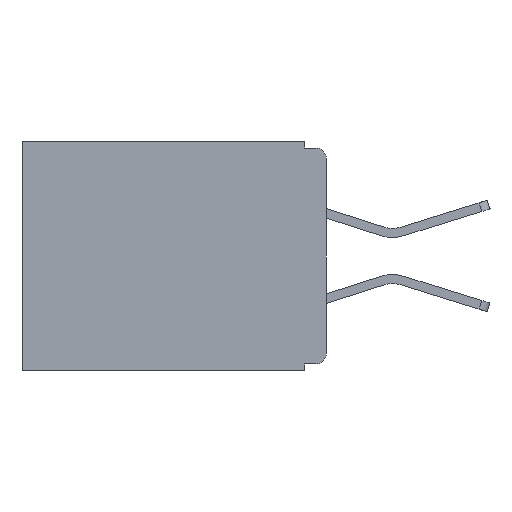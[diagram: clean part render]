
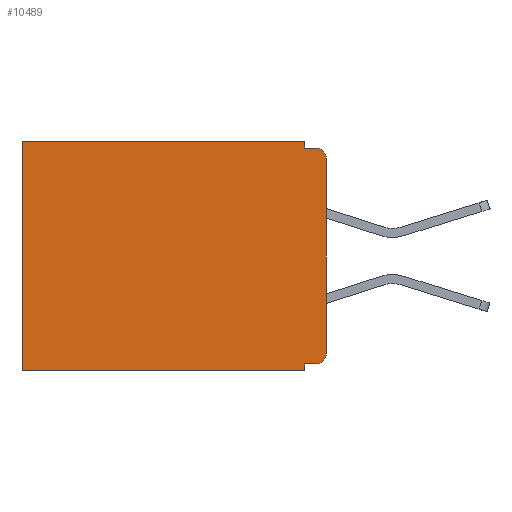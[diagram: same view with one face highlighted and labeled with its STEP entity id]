
A CAD part, left-side view. The second image highlights one B-rep face of the part: STEP entity #10489.
In plain terms, the highlighted planar face has unit normal (-1, 0, 0).
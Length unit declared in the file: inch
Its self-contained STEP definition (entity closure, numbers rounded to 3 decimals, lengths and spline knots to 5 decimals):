
#35 = VECTOR ( 'NONE', #5885, 39.37008 ) ;
#160 = EDGE_CURVE ( 'NONE', #6689, #9604, #744, .T. ) ;
#280 = CARTESIAN_POINT ( 'NONE',  ( 0.3, 0.031, -0.33 ) ) ;
#284 = ORIENTED_EDGE ( 'NONE', *, *, #694, .T. ) ;
#452 = VERTEX_POINT ( 'NONE', #13264 ) ;
#694 = EDGE_CURVE ( 'NONE', #452, #7662, #9821, .T. ) ;
#744 = LINE ( 'NONE', #280, #10207 ) ;
#772 = VECTOR ( 'NONE', #11210, 39.37008 ) ;
#854 = ORIENTED_EDGE ( 'NONE', *, *, #4215, .T. ) ;
#912 = DIRECTION ( 'NONE',  ( -1., 0., 0. ) ) ;
#950 = AXIS2_PLACEMENT_3D ( 'NONE', #11821, #8310, #1237 ) ;
#1017 = CARTESIAN_POINT ( 'NONE',  ( 0.3, 0., -0.33 ) ) ;
#1151 = LINE ( 'NONE', #1743, #772 ) ;
#1237 = DIRECTION ( 'NONE',  ( 0., 0., -1. ) ) ;
#1316 = CARTESIAN_POINT ( 'NONE',  ( 0.3, 0.437, 0. ) ) ;
#1378 = CARTESIAN_POINT ( 'NONE',  ( 0.3, 0., -0.025 ) ) ;
#1399 = VERTEX_POINT ( 'NONE', #8442 ) ;
#1604 = ORIENTED_EDGE ( 'NONE', *, *, #6825, .F. ) ;
#1619 = EDGE_CURVE ( 'NONE', #11748, #8068, #4103, .T. ) ;
#1743 = CARTESIAN_POINT ( 'NONE',  ( 0.3, 0., -0.32 ) ) ;
#1780 = LINE ( 'NONE', #13964, #13871 ) ;
#2155 = DIRECTION ( 'NONE',  ( 0., 0., -1. ) ) ;
#3025 = EDGE_CURVE ( 'NONE', #9604, #1399, #12511, .T. ) ;
#3147 = VECTOR ( 'NONE', #4138, 39.37008 ) ;
#3318 = AXIS2_PLACEMENT_3D ( 'NONE', #4435, #912, #2155 ) ;
#3719 = VECTOR ( 'NONE', #7602, 39.37008 ) ;
#3904 = CARTESIAN_POINT ( 'NONE',  ( 0.3, 0.031, -0.32 ) ) ;
#3993 = VERTEX_POINT ( 'NONE', #1316 ) ;
#4103 = LINE ( 'NONE', #7633, #13071 ) ;
#4138 = DIRECTION ( 'NONE',  ( 0., 1., 0. ) ) ;
#4215 = EDGE_CURVE ( 'NONE', #12995, #3993, #1780, .T. ) ;
#4247 = EDGE_CURVE ( 'NONE', #14159, #8068, #7720, .T. ) ;
#4289 = FACE_OUTER_BOUND ( 'NONE', #14512, .T. ) ;
#4435 = CARTESIAN_POINT ( 'NONE',  ( 0.3, 0.015, -0.025 ) ) ;
#4791 = CARTESIAN_POINT ( 'NONE',  ( 0.3, 0.015, -0.305 ) ) ;
#4856 = CARTESIAN_POINT ( 'NONE',  ( 0.3, 0.031, -0.01 ) ) ;
#4894 = VECTOR ( 'NONE', #7473, 39.37008 ) ;
#5332 = DIRECTION ( 'NONE',  ( 0., 0., -1. ) ) ;
#5620 = LINE ( 'NONE', #14393, #4894 ) ;
#5885 = DIRECTION ( 'NONE',  ( 0., 0., -1. ) ) ;
#6000 = LINE ( 'NONE', #12893, #35 ) ;
#6231 = ORIENTED_EDGE ( 'NONE', *, *, #7115, .T. ) ;
#6270 = CARTESIAN_POINT ( 'NONE',  ( 0.3, 0.031, -0.33 ) ) ;
#6432 = CARTESIAN_POINT ( 'NONE',  ( 0.3, 0.031, 0. ) ) ;
#6586 = ORIENTED_EDGE ( 'NONE', *, *, #9684, .F. ) ;
#6689 = VERTEX_POINT ( 'NONE', #3904 ) ;
#6709 = LINE ( 'NONE', #6432, #3719 ) ;
#6825 = EDGE_CURVE ( 'NONE', #452, #6689, #1151, .T. ) ;
#7105 = PLANE ( 'NONE',  #950 ) ;
#7115 = EDGE_CURVE ( 'NONE', #3993, #1399, #6000, .T. ) ;
#7275 = ORIENTED_EDGE ( 'NONE', *, *, #160, .F. ) ;
#7473 = DIRECTION ( 'NONE',  ( 0., 0., -1. ) ) ;
#7602 = DIRECTION ( 'NONE',  ( 0., 0., -1. ) ) ;
#7633 = CARTESIAN_POINT ( 'NONE',  ( 0.3, 0., -0.01 ) ) ;
#7662 = VERTEX_POINT ( 'NONE', #9455 ) ;
#7720 = CIRCLE ( 'NONE', #3318, 0.015 ) ;
#7861 = ORIENTED_EDGE ( 'NONE', *, *, #8957, .F. ) ;
#8068 = VERTEX_POINT ( 'NONE', #14982 ) ;
#8310 = DIRECTION ( 'NONE',  ( 1., 0., 0. ) ) ;
#8442 = CARTESIAN_POINT ( 'NONE',  ( 0.3, 0.437, -0.33 ) ) ;
#8957 = EDGE_CURVE ( 'NONE', #14159, #7662, #5620, .T. ) ;
#9455 = CARTESIAN_POINT ( 'NONE',  ( 0.3, 0., -0.305 ) ) ;
#9557 = DIRECTION ( 'NONE',  ( 0., 1., 0. ) ) ;
#9604 = VERTEX_POINT ( 'NONE', #6270 ) ;
#9684 = EDGE_CURVE ( 'NONE', #12995, #11748, #6709, .T. ) ;
#9744 = ORIENTED_EDGE ( 'NONE', *, *, #3025, .F. ) ;
#9821 = CIRCLE ( 'NONE', #11335, 0.015 ) ;
#10207 = VECTOR ( 'NONE', #5332, 39.37008 ) ;
#10489 = ADVANCED_FACE ( 'NONE', ( #4289 ), #7105, .F. ) ;
#10717 = DIRECTION ( 'NONE',  ( -1., 0., 0. ) ) ;
#11004 = CARTESIAN_POINT ( 'NONE',  ( 0.3, 0.031, 0. ) ) ;
#11196 = ORIENTED_EDGE ( 'NONE', *, *, #1619, .F. ) ;
#11210 = DIRECTION ( 'NONE',  ( 0., 1., 0. ) ) ;
#11335 = AXIS2_PLACEMENT_3D ( 'NONE', #4791, #10717, #11880 ) ;
#11748 = VERTEX_POINT ( 'NONE', #4856 ) ;
#11821 = CARTESIAN_POINT ( 'NONE',  ( 0.3, 0., -0.33 ) ) ;
#11880 = DIRECTION ( 'NONE',  ( 0., 0., -1. ) ) ;
#12376 = DIRECTION ( 'NONE',  ( 0., -1., 0. ) ) ;
#12511 = LINE ( 'NONE', #1017, #3147 ) ;
#12893 = CARTESIAN_POINT ( 'NONE',  ( 0.3, 0.437, -0.33 ) ) ;
#12995 = VERTEX_POINT ( 'NONE', #11004 ) ;
#13071 = VECTOR ( 'NONE', #12376, 39.37008 ) ;
#13264 = CARTESIAN_POINT ( 'NONE',  ( 0.3, 0.015, -0.32 ) ) ;
#13325 = ORIENTED_EDGE ( 'NONE', *, *, #4247, .T. ) ;
#13871 = VECTOR ( 'NONE', #9557, 39.37008 ) ;
#13964 = CARTESIAN_POINT ( 'NONE',  ( 0.3, 0., 0. ) ) ;
#14159 = VERTEX_POINT ( 'NONE', #1378 ) ;
#14393 = CARTESIAN_POINT ( 'NONE',  ( 0.3, 0., -0.33 ) ) ;
#14512 = EDGE_LOOP ( 'NONE', ( #7861, #13325, #11196, #6586, #854, #6231, #9744, #7275, #1604, #284 ) ) ;
#14982 = CARTESIAN_POINT ( 'NONE',  ( 0.3, 0.015, -0.01 ) ) ;
